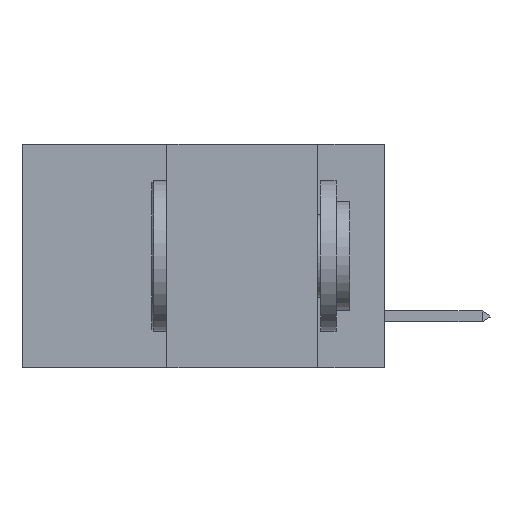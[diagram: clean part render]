
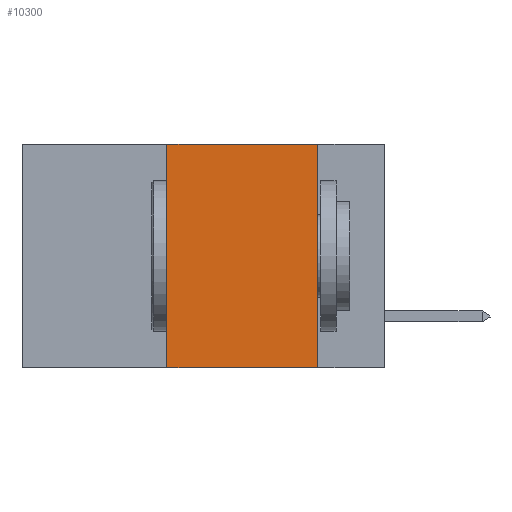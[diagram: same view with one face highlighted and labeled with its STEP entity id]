
A CAD part, left-side view. The second image highlights one B-rep face of the part: STEP entity #10300.
In plain terms, the highlighted planar face has unit normal (-1, 0, 0).
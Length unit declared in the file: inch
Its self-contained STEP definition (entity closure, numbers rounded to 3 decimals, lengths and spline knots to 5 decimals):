
#3055 = EDGE_CURVE ( 'NONE', #14915, #14050, #5382, .T. ) ;
#3889 = DIRECTION ( 'NONE',  ( 0., -1., 0. ) ) ;
#3922 = EDGE_LOOP ( 'NONE', ( #4361, #14439, #18251, #7136 ) ) ;
#4361 = ORIENTED_EDGE ( 'NONE', *, *, #3055, .F. ) ;
#4383 = LINE ( 'NONE', #14660, #28825 ) ;
#5027 = FACE_OUTER_BOUND ( 'NONE', #3922, .T. ) ;
#5382 = LINE ( 'NONE', #20562, #18706 ) ;
#6088 = CARTESIAN_POINT ( 'NONE',  ( 0., 0.11, 0. ) ) ;
#7136 = ORIENTED_EDGE ( 'NONE', *, *, #26608, .T. ) ;
#7617 = VECTOR ( 'NONE', #3889, 39.37008 ) ;
#7928 = CARTESIAN_POINT ( 'NONE',  ( 0., 0.11, -0.37 ) ) ;
#10300 = ADVANCED_FACE ( 'NONE', ( #5027 ), #13841, .F. ) ;
#13188 = LINE ( 'NONE', #22801, #7617 ) ;
#13841 = PLANE ( 'NONE',  #19049 ) ;
#14050 = VERTEX_POINT ( 'NONE', #7928 ) ;
#14439 = ORIENTED_EDGE ( 'NONE', *, *, #30657, .F. ) ;
#14660 = CARTESIAN_POINT ( 'NONE',  ( 0., 0.6, 0. ) ) ;
#14858 = EDGE_CURVE ( 'NONE', #17943, #15086, #30388, .T. ) ;
#14915 = VERTEX_POINT ( 'NONE', #6088 ) ;
#15086 = VERTEX_POINT ( 'NONE', #15206 ) ;
#15206 = CARTESIAN_POINT ( 'NONE',  ( 0., 0.36, 0. ) ) ;
#17943 = VERTEX_POINT ( 'NONE', #29586 ) ;
#18251 = ORIENTED_EDGE ( 'NONE', *, *, #14858, .F. ) ;
#18706 = VECTOR ( 'NONE', #23140, 39.37008 ) ;
#19049 = AXIS2_PLACEMENT_3D ( 'NONE', #23322, #20945, #25826 ) ;
#19113 = DIRECTION ( 'NONE',  ( 0., -1., 0. ) ) ;
#20562 = CARTESIAN_POINT ( 'NONE',  ( 0., 0.11, 0. ) ) ;
#20945 = DIRECTION ( 'NONE',  ( 1., 0., 0. ) ) ;
#22801 = CARTESIAN_POINT ( 'NONE',  ( 0., 0.6, -0.37 ) ) ;
#23140 = DIRECTION ( 'NONE',  ( 0., 0., -1. ) ) ;
#23322 = CARTESIAN_POINT ( 'NONE',  ( 0., 0.6, 0. ) ) ;
#24585 = CARTESIAN_POINT ( 'NONE',  ( 0., 0.36, 0. ) ) ;
#25826 = DIRECTION ( 'NONE',  ( 0., 0., -1. ) ) ;
#26608 = EDGE_CURVE ( 'NONE', #17943, #14050, #13188, .T. ) ;
#28173 = VECTOR ( 'NONE', #29400, 39.37008 ) ;
#28825 = VECTOR ( 'NONE', #19113, 39.37008 ) ;
#29400 = DIRECTION ( 'NONE',  ( 0., 0., 1. ) ) ;
#29586 = CARTESIAN_POINT ( 'NONE',  ( 0., 0.36, -0.37 ) ) ;
#30388 = LINE ( 'NONE', #24585, #28173 ) ;
#30657 = EDGE_CURVE ( 'NONE', #15086, #14915, #4383, .T. ) ;
